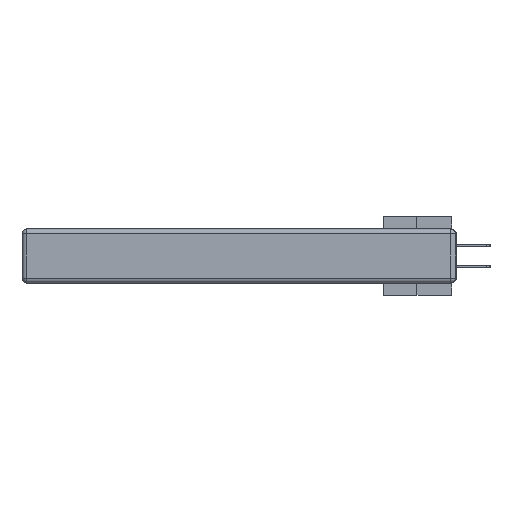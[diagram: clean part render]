
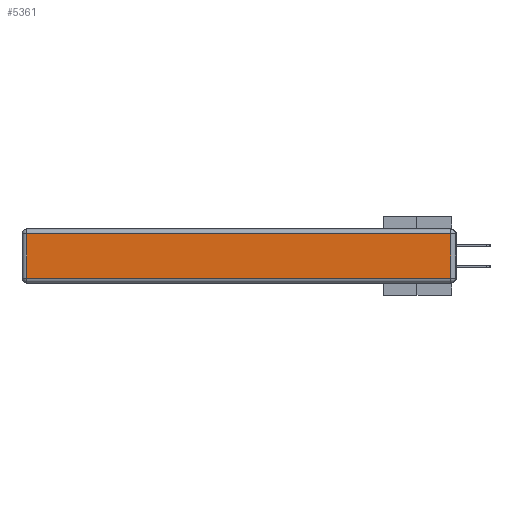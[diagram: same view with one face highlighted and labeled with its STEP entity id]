
A CAD part, left-side view. The second image highlights one B-rep face of the part: STEP entity #5361.
In plain terms, the highlighted planar face has unit normal (-1, 0, 0).
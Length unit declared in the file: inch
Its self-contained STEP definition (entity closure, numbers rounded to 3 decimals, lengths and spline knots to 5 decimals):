
#9 = CARTESIAN_POINT ( 'NONE',  ( 0., 2.72, -0.343 ) ) ;
#936 = LINE ( 'NONE', #9201, #13029 ) ;
#1533 = LINE ( 'NONE', #14743, #32635 ) ;
#1696 = VERTEX_POINT ( 'NONE', #41293 ) ;
#1744 = PLANE ( 'NONE',  #42044 ) ;
#2551 = FACE_OUTER_BOUND ( 'NONE', #29837, .T. ) ;
#5361 = ADVANCED_FACE ( 'NONE', ( #2551 ), #1744, .T. ) ;
#7630 = CARTESIAN_POINT ( 'NONE',  ( 0., 0.03, -0.03 ) ) ;
#9201 = CARTESIAN_POINT ( 'NONE',  ( 0., 0.03, -0.343 ) ) ;
#12601 = DIRECTION ( 'NONE',  ( -1., 0., 0. ) ) ;
#13029 = VECTOR ( 'NONE', #33742, 39.37008 ) ;
#14402 = EDGE_CURVE ( 'NONE', #22878, #26501, #35721, .T. ) ;
#14743 = CARTESIAN_POINT ( 'NONE',  ( 0., 2.75, -0.03 ) ) ;
#16148 = CARTESIAN_POINT ( 'NONE',  ( 0., 2.72, -0.03 ) ) ;
#16726 = DIRECTION ( 'NONE',  ( 0., -1., 0. ) ) ;
#20381 = ORIENTED_EDGE ( 'NONE', *, *, #25266, .T. ) ;
#20527 = CARTESIAN_POINT ( 'NONE',  ( 0., 0., -0.313 ) ) ;
#22589 = VERTEX_POINT ( 'NONE', #7630 ) ;
#22878 = VERTEX_POINT ( 'NONE', #16148 ) ;
#23151 = VECTOR ( 'NONE', #38621, 39.37008 ) ;
#24002 = VECTOR ( 'NONE', #16726, 39.37008 ) ;
#24177 = ORIENTED_EDGE ( 'NONE', *, *, #25499, .T. ) ;
#25266 = EDGE_CURVE ( 'NONE', #1696, #22589, #936, .T. ) ;
#25499 = EDGE_CURVE ( 'NONE', #22589, #22878, #1533, .T. ) ;
#26501 = VERTEX_POINT ( 'NONE', #28731 ) ;
#27284 = ORIENTED_EDGE ( 'NONE', *, *, #34597, .T. ) ;
#28731 = CARTESIAN_POINT ( 'NONE',  ( 0., 2.72, -0.313 ) ) ;
#29837 = EDGE_LOOP ( 'NONE', ( #27284, #20381, #24177, #38395 ) ) ;
#32635 = VECTOR ( 'NONE', #39176, 39.37008 ) ;
#33742 = DIRECTION ( 'NONE',  ( 0., 0., 1. ) ) ;
#34597 = EDGE_CURVE ( 'NONE', #26501, #1696, #43129, .T. ) ;
#35721 = LINE ( 'NONE', #9, #23151 ) ;
#36531 = DIRECTION ( 'NONE',  ( 0., 0., 1. ) ) ;
#38395 = ORIENTED_EDGE ( 'NONE', *, *, #14402, .T. ) ;
#38621 = DIRECTION ( 'NONE',  ( 0., 0., -1. ) ) ;
#39176 = DIRECTION ( 'NONE',  ( 0., 1., 0. ) ) ;
#41293 = CARTESIAN_POINT ( 'NONE',  ( 0., 0.03, -0.313 ) ) ;
#42044 = AXIS2_PLACEMENT_3D ( 'NONE', #43848, #12601, #36531 ) ;
#43129 = LINE ( 'NONE', #20527, #24002 ) ;
#43848 = CARTESIAN_POINT ( 'NONE',  ( 0., 0., -0.343 ) ) ;
